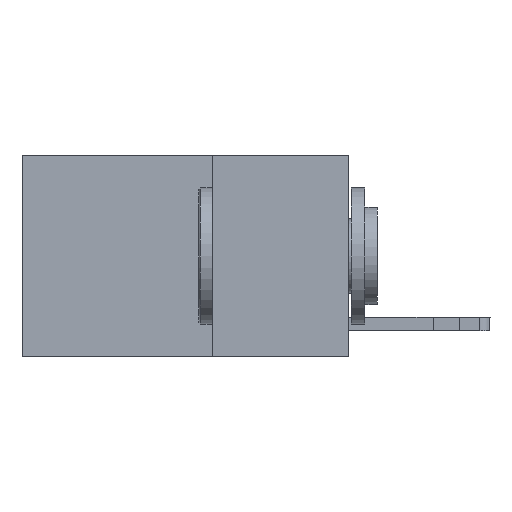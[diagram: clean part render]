
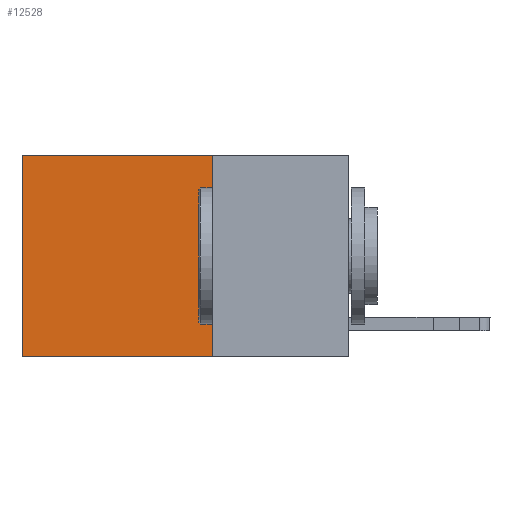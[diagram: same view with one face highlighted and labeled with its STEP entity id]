
A CAD part, left-side view. The second image highlights one B-rep face of the part: STEP entity #12528.
In plain terms, the highlighted planar face has unit normal (-1, 0, 0).
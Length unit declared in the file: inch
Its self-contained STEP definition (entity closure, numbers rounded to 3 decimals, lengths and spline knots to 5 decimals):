
#22 = CARTESIAN_POINT ( 'NONE',  ( 0.2625, 0.6, 0. ) ) ;
#915 = VECTOR ( 'NONE', #14003, 39.37008 ) ;
#1050 = DIRECTION ( 'NONE',  ( 0., 0., -1. ) ) ;
#1164 = CARTESIAN_POINT ( 'NONE',  ( 0.2625, 0.6, 0. ) ) ;
#1755 = ORIENTED_EDGE ( 'NONE', *, *, #3933, .T. ) ;
#1798 = EDGE_CURVE ( 'NONE', #8636, #5015, #12949, .T. ) ;
#1918 = CARTESIAN_POINT ( 'NONE',  ( 0.2625, 0.25, 0. ) ) ;
#2180 = LINE ( 'NONE', #7162, #4200 ) ;
#2694 = DIRECTION ( 'NONE',  ( 0., 0., -1. ) ) ;
#3252 = DIRECTION ( 'NONE',  ( 0., 0., -1. ) ) ;
#3327 = CARTESIAN_POINT ( 'NONE',  ( 0.2625, 0.25, -0.37 ) ) ;
#3855 = ORIENTED_EDGE ( 'NONE', *, *, #9244, .F. ) ;
#3933 = EDGE_CURVE ( 'NONE', #5015, #4549, #13479, .T. ) ;
#4200 = VECTOR ( 'NONE', #1050, 39.37008 ) ;
#4255 = ORIENTED_EDGE ( 'NONE', *, *, #1798, .T. ) ;
#4549 = VERTEX_POINT ( 'NONE', #15064 ) ;
#5015 = VERTEX_POINT ( 'NONE', #22 ) ;
#5310 = VECTOR ( 'NONE', #2694, 39.37008 ) ;
#6010 = EDGE_LOOP ( 'NONE', ( #1755, #3855, #9799, #4255 ) ) ;
#6154 = CARTESIAN_POINT ( 'NONE',  ( 0.2625, 0.25, -0.37 ) ) ;
#6213 = VERTEX_POINT ( 'NONE', #3327 ) ;
#7162 = CARTESIAN_POINT ( 'NONE',  ( 0.2625, 0.25, 0. ) ) ;
#8636 = VERTEX_POINT ( 'NONE', #10931 ) ;
#9244 = EDGE_CURVE ( 'NONE', #6213, #4549, #10997, .T. ) ;
#9331 = CARTESIAN_POINT ( 'NONE',  ( 0.2625, 0.25, 0. ) ) ;
#9479 = EDGE_CURVE ( 'NONE', #8636, #6213, #2180, .T. ) ;
#9516 = AXIS2_PLACEMENT_3D ( 'NONE', #9331, #14266, #3252 ) ;
#9799 = ORIENTED_EDGE ( 'NONE', *, *, #9479, .F. ) ;
#10631 = PLANE ( 'NONE',  #9516 ) ;
#10931 = CARTESIAN_POINT ( 'NONE',  ( 0.2625, 0.25, 0. ) ) ;
#10997 = LINE ( 'NONE', #6154, #15895 ) ;
#12528 = ADVANCED_FACE ( 'NONE', ( #15456 ), #10631, .F. ) ;
#12949 = LINE ( 'NONE', #1918, #915 ) ;
#13479 = LINE ( 'NONE', #1164, #5310 ) ;
#13863 = DIRECTION ( 'NONE',  ( 0., 1., 0. ) ) ;
#14003 = DIRECTION ( 'NONE',  ( 0., 1., 0. ) ) ;
#14266 = DIRECTION ( 'NONE',  ( 1., 0., 0. ) ) ;
#15064 = CARTESIAN_POINT ( 'NONE',  ( 0.2625, 0.6, -0.37 ) ) ;
#15456 = FACE_OUTER_BOUND ( 'NONE', #6010, .T. ) ;
#15895 = VECTOR ( 'NONE', #13863, 39.37008 ) ;
